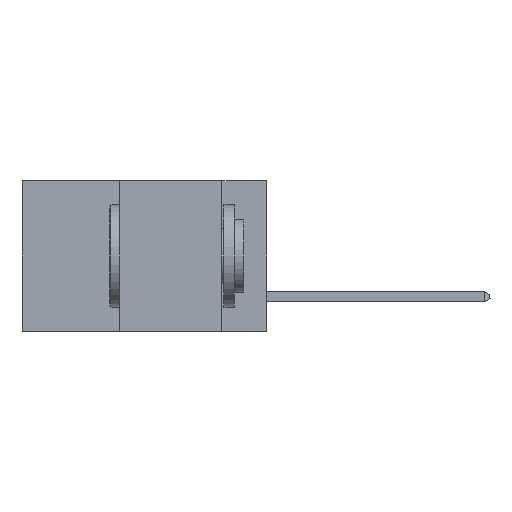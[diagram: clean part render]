
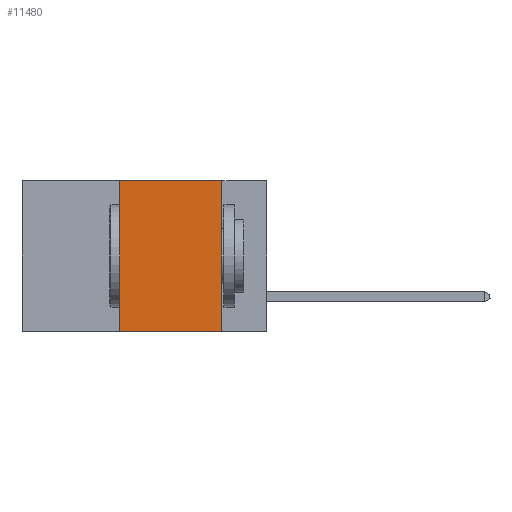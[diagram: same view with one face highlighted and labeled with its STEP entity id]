
A CAD part, left-side view. The second image highlights one B-rep face of the part: STEP entity #11480.
In plain terms, the highlighted planar face has unit normal (-1, 0, 0).
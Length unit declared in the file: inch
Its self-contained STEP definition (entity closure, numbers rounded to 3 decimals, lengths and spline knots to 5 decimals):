
#173 = ORIENTED_EDGE ( 'NONE', *, *, #21500, .F. ) ;
#782 = CARTESIAN_POINT ( 'NONE',  ( 0., 0.36, 0. ) ) ;
#909 = VECTOR ( 'NONE', #21258, 39.37008 ) ;
#1283 = ORIENTED_EDGE ( 'NONE', *, *, #14189, .F. ) ;
#3121 = CARTESIAN_POINT ( 'NONE',  ( 0., 0.11, -0.37 ) ) ;
#3137 = CARTESIAN_POINT ( 'NONE',  ( 0., 0.6, 0. ) ) ;
#4722 = EDGE_LOOP ( 'NONE', ( #13715, #173, #1283, #6620 ) ) ;
#4925 = DIRECTION ( 'NONE',  ( 0., 0., -1. ) ) ;
#5081 = DIRECTION ( 'NONE',  ( 0., 0., 1. ) ) ;
#5849 = EDGE_CURVE ( 'NONE', #7086, #18286, #17783, .T. ) ;
#6620 = ORIENTED_EDGE ( 'NONE', *, *, #5849, .T. ) ;
#7018 = CARTESIAN_POINT ( 'NONE',  ( 0., 0.11, 0. ) ) ;
#7086 = VERTEX_POINT ( 'NONE', #18449 ) ;
#7663 = FACE_OUTER_BOUND ( 'NONE', #4722, .T. ) ;
#8323 = CARTESIAN_POINT ( 'NONE',  ( 0., 0.11, 0. ) ) ;
#8371 = VECTOR ( 'NONE', #20756, 39.37008 ) ;
#8649 = CARTESIAN_POINT ( 'NONE',  ( 0., 0.36, 0. ) ) ;
#10016 = VECTOR ( 'NONE', #5081, 39.37008 ) ;
#10562 = LINE ( 'NONE', #8649, #10016 ) ;
#10982 = CARTESIAN_POINT ( 'NONE',  ( 0., 0.6, 0. ) ) ;
#11480 = ADVANCED_FACE ( 'NONE', ( #7663 ), #20391, .F. ) ;
#12757 = VECTOR ( 'NONE', #16898, 39.37008 ) ;
#13178 = VERTEX_POINT ( 'NONE', #782 ) ;
#13715 = ORIENTED_EDGE ( 'NONE', *, *, #14246, .F. ) ;
#14189 = EDGE_CURVE ( 'NONE', #7086, #13178, #10562, .T. ) ;
#14246 = EDGE_CURVE ( 'NONE', #18815, #18286, #18036, .T. ) ;
#15204 = CARTESIAN_POINT ( 'NONE',  ( 0., 0.6, -0.37 ) ) ;
#15401 = DIRECTION ( 'NONE',  ( 1., 0., 0. ) ) ;
#16898 = DIRECTION ( 'NONE',  ( 0., -1., 0. ) ) ;
#16983 = AXIS2_PLACEMENT_3D ( 'NONE', #3137, #15401, #4925 ) ;
#17783 = LINE ( 'NONE', #15204, #12757 ) ;
#18036 = LINE ( 'NONE', #7018, #8371 ) ;
#18286 = VERTEX_POINT ( 'NONE', #3121 ) ;
#18449 = CARTESIAN_POINT ( 'NONE',  ( 0., 0.36, -0.37 ) ) ;
#18815 = VERTEX_POINT ( 'NONE', #8323 ) ;
#19453 = LINE ( 'NONE', #10982, #909 ) ;
#20391 = PLANE ( 'NONE',  #16983 ) ;
#20756 = DIRECTION ( 'NONE',  ( 0., 0., -1. ) ) ;
#21258 = DIRECTION ( 'NONE',  ( 0., -1., 0. ) ) ;
#21500 = EDGE_CURVE ( 'NONE', #13178, #18815, #19453, .T. ) ;
